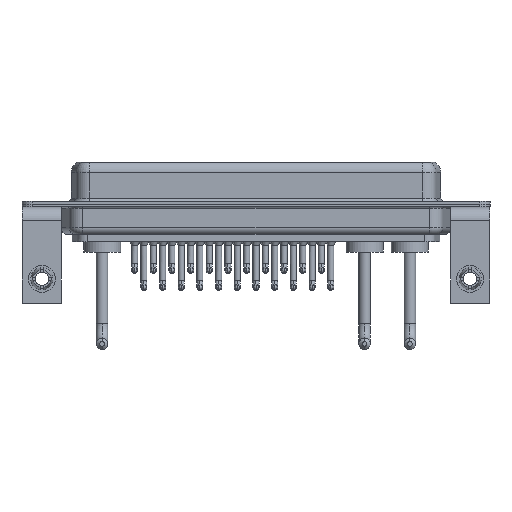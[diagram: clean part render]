
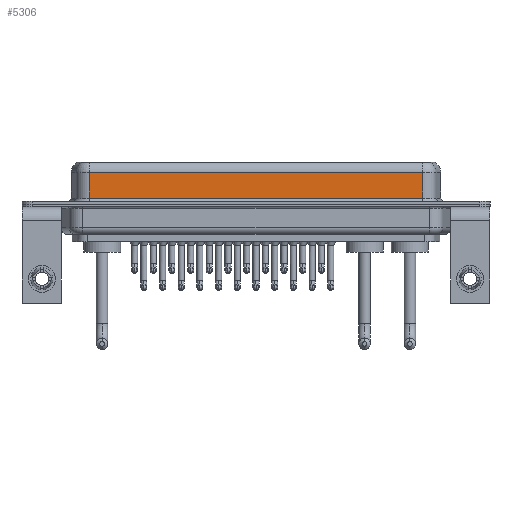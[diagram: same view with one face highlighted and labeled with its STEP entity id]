
A CAD part, front view. The second image highlights one B-rep face of the part: STEP entity #5306.
In plain terms, the highlighted planar face has unit normal (0, -1, 0).
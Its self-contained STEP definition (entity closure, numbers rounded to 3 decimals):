
#110 = VECTOR ( 'NONE', #14017, 1000. ) ;
#283 = CARTESIAN_POINT ( 'NONE',  ( 56.462, -3.95, 4.65 ) ) ;
#552 = CARTESIAN_POINT ( 'NONE',  ( 56.462, -3.95, 0.9 ) ) ;
#1577 = CARTESIAN_POINT ( 'NONE',  ( 56.462, -3.95, 6.4 ) ) ;
#2927 = EDGE_CURVE ( 'NONE', #17223, #3901, #13891, .T. ) ;
#3901 = VERTEX_POINT ( 'NONE', #4029 ) ;
#4029 = CARTESIAN_POINT ( 'NONE',  ( 7.038, -3.95, 0.9 ) ) ;
#4044 = ORIENTED_EDGE ( 'NONE', *, *, #11294, .F. ) ;
#4245 = CARTESIAN_POINT ( 'NONE',  ( 56.462, -3.95, 6.4 ) ) ;
#4969 = VERTEX_POINT ( 'NONE', #7037 ) ;
#5306 = ADVANCED_FACE ( 'NONE', ( #14577 ), #10586, .F. ) ;
#6570 = EDGE_CURVE ( 'NONE', #3901, #13412, #12461, .T. ) ;
#7037 = CARTESIAN_POINT ( 'NONE',  ( 56.462, -3.95, 4.65 ) ) ;
#7327 = VECTOR ( 'NONE', #21991, 1000. ) ;
#8473 = DIRECTION ( 'NONE',  ( 0., 1., 0. ) ) ;
#10323 = LINE ( 'NONE', #283, #12772 ) ;
#10586 = PLANE ( 'NONE',  #17850 ) ;
#10928 = EDGE_CURVE ( 'NONE', #4969, #17223, #10323, .T. ) ;
#11294 = EDGE_CURVE ( 'NONE', #4969, #13412, #13750, .T. ) ;
#12461 = LINE ( 'NONE', #552, #14237 ) ;
#12772 = VECTOR ( 'NONE', #14054, 1000. ) ;
#13392 = CARTESIAN_POINT ( 'NONE',  ( 56.462, -3.95, 0.9 ) ) ;
#13412 = VERTEX_POINT ( 'NONE', #13392 ) ;
#13508 = ORIENTED_EDGE ( 'NONE', *, *, #10928, .T. ) ;
#13750 = LINE ( 'NONE', #1577, #110 ) ;
#13890 = CARTESIAN_POINT ( 'NONE',  ( 7.038, -3.95, 4.65 ) ) ;
#13891 = LINE ( 'NONE', #18157, #7327 ) ;
#14017 = DIRECTION ( 'NONE',  ( 0., 0., -1. ) ) ;
#14054 = DIRECTION ( 'NONE',  ( -1., 0., 0. ) ) ;
#14237 = VECTOR ( 'NONE', #20822, 1000. ) ;
#14577 = FACE_OUTER_BOUND ( 'NONE', #20180, .T. ) ;
#16253 = ORIENTED_EDGE ( 'NONE', *, *, #6570, .T. ) ;
#17223 = VERTEX_POINT ( 'NONE', #13890 ) ;
#17850 = AXIS2_PLACEMENT_3D ( 'NONE', #4245, #8473, #24398 ) ;
#18157 = CARTESIAN_POINT ( 'NONE',  ( 7.038, -3.95, 6.4 ) ) ;
#20180 = EDGE_LOOP ( 'NONE', ( #4044, #13508, #25816, #16253 ) ) ;
#20822 = DIRECTION ( 'NONE',  ( 1., 0., 0. ) ) ;
#21991 = DIRECTION ( 'NONE',  ( 0., 0., -1. ) ) ;
#24398 = DIRECTION ( 'NONE',  ( 0., 0., 1. ) ) ;
#25816 = ORIENTED_EDGE ( 'NONE', *, *, #2927, .T. ) ;
